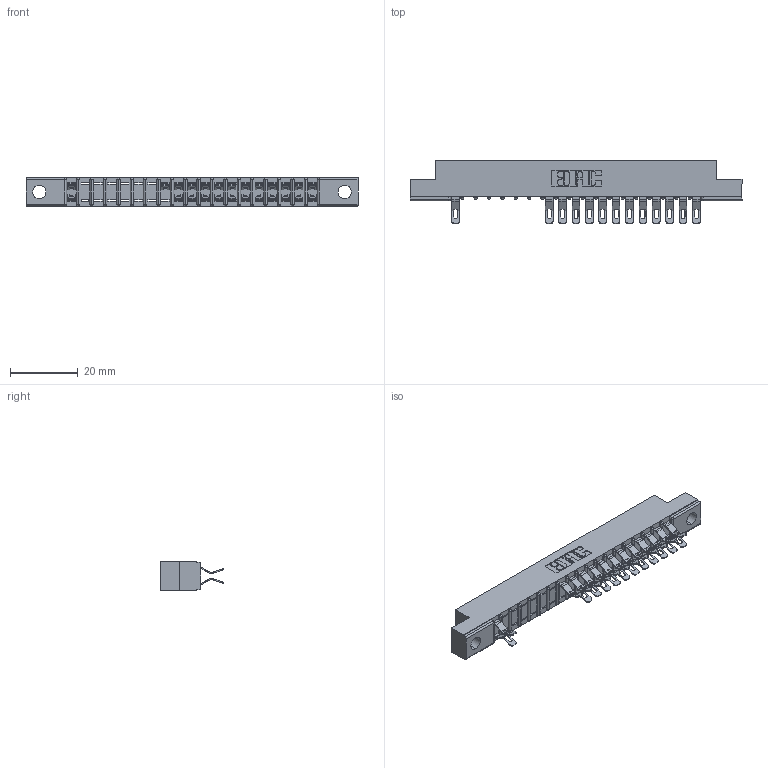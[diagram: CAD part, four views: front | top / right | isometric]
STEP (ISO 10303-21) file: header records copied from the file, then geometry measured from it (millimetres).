
FILE_DESCRIPTION (( 'STEP AP203' ), '1' );
FILE_NAME ('307-038-555-204.STEP', '2018-08-05T11:55:59', ( '' ), ( '' ), 'SwSTEP 2.0', 'SolidWorks 2016', '' );
FILE_SCHEMA (( 'CONFIG_CONTROL_DESIGN' ));
Length unit declared in the file: inch
Products named in the file (3): 307 Part_.156 Dia Mounting Holes; 307-290-001_555; 307-038-555-204
Assembly tree (26 placements, depth 2):
  307-038-555-204
    307 Part_.156 Dia Mounting Holes
    307-290-001_555  x25
Bounding box: 98.3 x 18.75 x 8.71 mm (x, y, z)
Volume: 6230.3 mm3; surface area: 10153.7 mm2
Topology: 26 solids, 26 shells, 1807 faces, 5300 edges, 3444 vertices
Faces by surface type: plane 1012, cylinder 755, sphere 40
Entity records: 20271 total; most frequent: CARTESIAN_POINT 3388, ORIENTED_EDGE 3368, DIRECTION 3314, EDGE_CURVE 1684, LINE 1278, VECTOR 1278, VERTEX_POINT 1092, AXIS2_PLACEMENT_3D 1018
